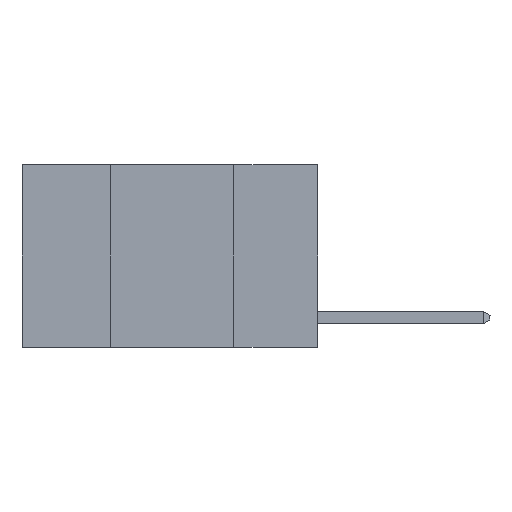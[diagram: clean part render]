
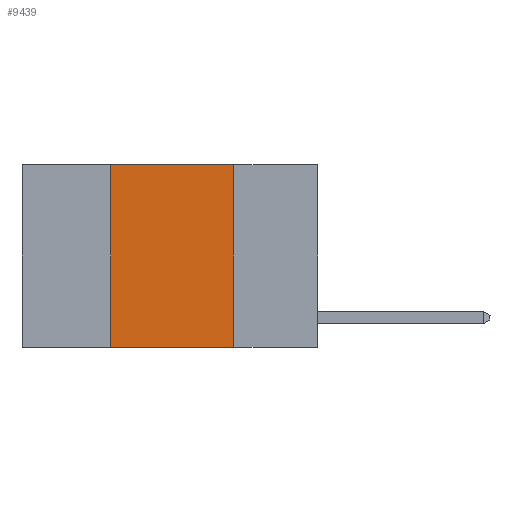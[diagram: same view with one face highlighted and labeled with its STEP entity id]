
A CAD part, left-side view. The second image highlights one B-rep face of the part: STEP entity #9439.
In plain terms, the highlighted planar face has unit normal (-1, 0, 0).
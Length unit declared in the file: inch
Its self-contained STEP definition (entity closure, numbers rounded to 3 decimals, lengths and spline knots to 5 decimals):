
#24 = EDGE_CURVE ( 'NONE', #5970, #5264, #5358, .T. ) ;
#607 = LINE ( 'NONE', #3622, #2030 ) ;
#1075 = FACE_OUTER_BOUND ( 'NONE', #8148, .T. ) ;
#1276 = LINE ( 'NONE', #2017, #5139 ) ;
#1333 = LINE ( 'NONE', #4468, #3266 ) ;
#1692 = ORIENTED_EDGE ( 'NONE', *, *, #5695, .F. ) ;
#1699 = CARTESIAN_POINT ( 'NONE',  ( 0., 0.17, 0. ) ) ;
#1847 = DIRECTION ( 'NONE',  ( 0., 0., -1. ) ) ;
#1910 = CARTESIAN_POINT ( 'NONE',  ( 0., 0.42, 0. ) ) ;
#2017 = CARTESIAN_POINT ( 'NONE',  ( 0., 0.6, 0. ) ) ;
#2030 = VECTOR ( 'NONE', #6563, 39.37008 ) ;
#2212 = CARTESIAN_POINT ( 'NONE',  ( 0., 0.42, -0.37 ) ) ;
#2542 = DIRECTION ( 'NONE',  ( 0., 0., -1. ) ) ;
#3266 = VECTOR ( 'NONE', #8158, 39.37008 ) ;
#3347 = ORIENTED_EDGE ( 'NONE', *, *, #8288, .F. ) ;
#3622 = CARTESIAN_POINT ( 'NONE',  ( 0., 0.6, -0.37 ) ) ;
#3981 = PLANE ( 'NONE',  #8432 ) ;
#4468 = CARTESIAN_POINT ( 'NONE',  ( 0., 0.42, 0. ) ) ;
#5139 = VECTOR ( 'NONE', #5718, 39.37008 ) ;
#5264 = VERTEX_POINT ( 'NONE', #7842 ) ;
#5358 = LINE ( 'NONE', #8343, #8580 ) ;
#5403 = EDGE_CURVE ( 'NONE', #7039, #5264, #607, .T. ) ;
#5695 = EDGE_CURVE ( 'NONE', #7659, #5970, #1276, .T. ) ;
#5718 = DIRECTION ( 'NONE',  ( 0., -1., 0. ) ) ;
#5970 = VERTEX_POINT ( 'NONE', #1699 ) ;
#6099 = ORIENTED_EDGE ( 'NONE', *, *, #5403, .T. ) ;
#6563 = DIRECTION ( 'NONE',  ( 0., -1., 0. ) ) ;
#7038 = DIRECTION ( 'NONE',  ( 1., 0., 0. ) ) ;
#7039 = VERTEX_POINT ( 'NONE', #2212 ) ;
#7659 = VERTEX_POINT ( 'NONE', #1910 ) ;
#7842 = CARTESIAN_POINT ( 'NONE',  ( 0., 0.17, -0.37 ) ) ;
#8148 = EDGE_LOOP ( 'NONE', ( #9573, #1692, #3347, #6099 ) ) ;
#8158 = DIRECTION ( 'NONE',  ( 0., 0., 1. ) ) ;
#8288 = EDGE_CURVE ( 'NONE', #7039, #7659, #1333, .T. ) ;
#8343 = CARTESIAN_POINT ( 'NONE',  ( 0., 0.17, 0. ) ) ;
#8432 = AXIS2_PLACEMENT_3D ( 'NONE', #9245, #7038, #1847 ) ;
#8580 = VECTOR ( 'NONE', #2542, 39.37008 ) ;
#9245 = CARTESIAN_POINT ( 'NONE',  ( 0., 0.6, 0. ) ) ;
#9439 = ADVANCED_FACE ( 'NONE', ( #1075 ), #3981, .F. ) ;
#9573 = ORIENTED_EDGE ( 'NONE', *, *, #24, .F. ) ;
